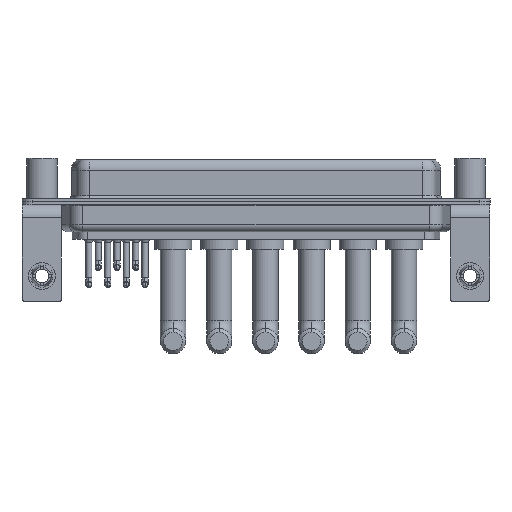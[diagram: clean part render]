
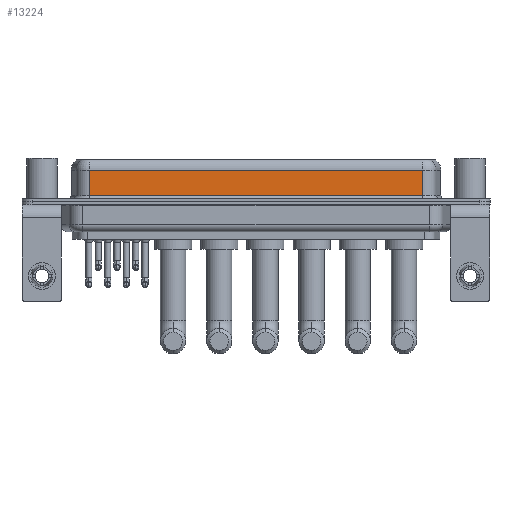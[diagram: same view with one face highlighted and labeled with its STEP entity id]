
A CAD part, front view. The second image highlights one B-rep face of the part: STEP entity #13224.
In plain terms, the highlighted planar face has unit normal (0, -1, 0).
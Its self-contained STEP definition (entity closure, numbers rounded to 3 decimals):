
#61 = LINE ( 'NONE', #377, #1064 ) ;
#377 = CARTESIAN_POINT ( 'NONE',  ( 56.462, -3.95, 4.65 ) ) ;
#915 = CARTESIAN_POINT ( 'NONE',  ( 56.462, -3.95, 0.9 ) ) ;
#1064 = VECTOR ( 'NONE', #13924, 1000. ) ;
#1102 = CARTESIAN_POINT ( 'NONE',  ( 7.038, -3.95, 0.9 ) ) ;
#2225 = VECTOR ( 'NONE', #11349, 1000. ) ;
#2910 = DIRECTION ( 'NONE',  ( 0., 1., 0. ) ) ;
#5432 = CARTESIAN_POINT ( 'NONE',  ( 56.462, -3.95, 4.65 ) ) ;
#5552 = CARTESIAN_POINT ( 'NONE',  ( 56.462, -3.95, 0.9 ) ) ;
#6742 = EDGE_CURVE ( 'NONE', #7200, #8828, #16133, .T. ) ;
#7123 = ORIENTED_EDGE ( 'NONE', *, *, #17455, .F. ) ;
#7200 = VERTEX_POINT ( 'NONE', #1102 ) ;
#7345 = VERTEX_POINT ( 'NONE', #9991 ) ;
#7909 = DIRECTION ( 'NONE',  ( 0., 0., 1. ) ) ;
#8306 = VECTOR ( 'NONE', #21439, 1000. ) ;
#8828 = VERTEX_POINT ( 'NONE', #5552 ) ;
#9543 = LINE ( 'NONE', #18184, #8306 ) ;
#9991 = CARTESIAN_POINT ( 'NONE',  ( 7.038, -3.95, 4.65 ) ) ;
#10143 = ORIENTED_EDGE ( 'NONE', *, *, #11113, .T. ) ;
#11113 = EDGE_CURVE ( 'NONE', #14419, #7345, #61, .T. ) ;
#11235 = VECTOR ( 'NONE', #15662, 1000. ) ;
#11349 = DIRECTION ( 'NONE',  ( 1., 0., 0. ) ) ;
#13224 = ADVANCED_FACE ( 'NONE', ( #18003 ), #21356, .F. ) ;
#13924 = DIRECTION ( 'NONE',  ( -1., 0., 0. ) ) ;
#14326 = LINE ( 'NONE', #17657, #11235 ) ;
#14419 = VERTEX_POINT ( 'NONE', #5432 ) ;
#15232 = AXIS2_PLACEMENT_3D ( 'NONE', #21809, #2910, #7909 ) ;
#15662 = DIRECTION ( 'NONE',  ( 0., 0., -1. ) ) ;
#15774 = EDGE_CURVE ( 'NONE', #7345, #7200, #14326, .T. ) ;
#16133 = LINE ( 'NONE', #915, #2225 ) ;
#17455 = EDGE_CURVE ( 'NONE', #14419, #8828, #9543, .T. ) ;
#17657 = CARTESIAN_POINT ( 'NONE',  ( 7.038, -3.95, 6.4 ) ) ;
#18003 = FACE_OUTER_BOUND ( 'NONE', #18110, .T. ) ;
#18110 = EDGE_LOOP ( 'NONE', ( #7123, #10143, #19918, #19546 ) ) ;
#18184 = CARTESIAN_POINT ( 'NONE',  ( 56.462, -3.95, 6.4 ) ) ;
#19546 = ORIENTED_EDGE ( 'NONE', *, *, #6742, .T. ) ;
#19918 = ORIENTED_EDGE ( 'NONE', *, *, #15774, .T. ) ;
#21356 = PLANE ( 'NONE',  #15232 ) ;
#21439 = DIRECTION ( 'NONE',  ( 0., 0., -1. ) ) ;
#21809 = CARTESIAN_POINT ( 'NONE',  ( 56.462, -3.95, 6.4 ) ) ;
